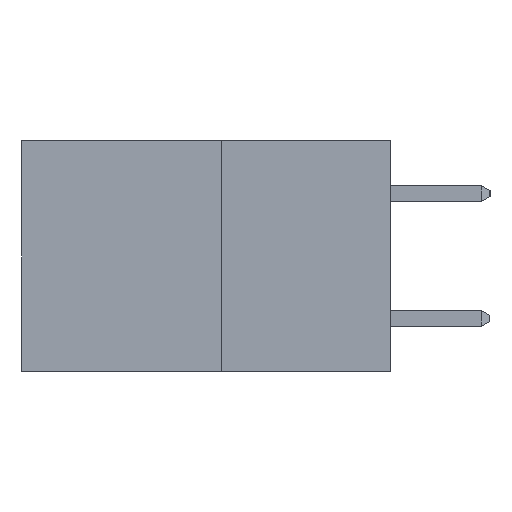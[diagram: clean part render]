
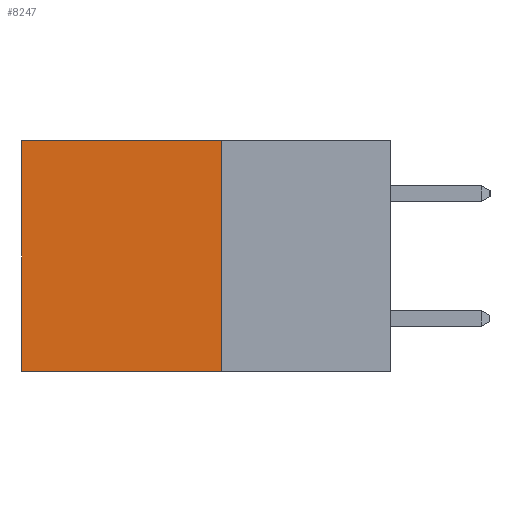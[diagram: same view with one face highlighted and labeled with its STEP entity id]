
A CAD part, left-side view. The second image highlights one B-rep face of the part: STEP entity #8247.
In plain terms, the highlighted planar face has unit normal (-1, 0, 0).
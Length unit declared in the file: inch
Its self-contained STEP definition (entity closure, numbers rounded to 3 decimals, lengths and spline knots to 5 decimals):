
#1089 = CARTESIAN_POINT ( 'NONE',  ( 0.277, 0.27, -0.37 ) ) ;
#1847 = FACE_OUTER_BOUND ( 'NONE', #21281, .T. ) ;
#1925 = EDGE_CURVE ( 'NONE', #2921, #8622, #12004, .T. ) ;
#2556 = EDGE_CURVE ( 'NONE', #2921, #6136, #14029, .T. ) ;
#2921 = VERTEX_POINT ( 'NONE', #9171 ) ;
#3023 = LINE ( 'NONE', #23436, #17572 ) ;
#3614 = DIRECTION ( 'NONE',  ( 1., 0., 0. ) ) ;
#3800 = DIRECTION ( 'NONE',  ( 0., 1., 0. ) ) ;
#3917 = VECTOR ( 'NONE', #9567, 39.37008 ) ;
#6136 = VERTEX_POINT ( 'NONE', #6301 ) ;
#6301 = CARTESIAN_POINT ( 'NONE',  ( 0.277, 0.59, 0. ) ) ;
#6983 = VECTOR ( 'NONE', #17974, 39.37008 ) ;
#7414 = VERTEX_POINT ( 'NONE', #19137 ) ;
#8247 = ADVANCED_FACE ( 'NONE', ( #1847 ), #24306, .F. ) ;
#8622 = VERTEX_POINT ( 'NONE', #14500 ) ;
#9171 = CARTESIAN_POINT ( 'NONE',  ( 0.277, 0.27, 0. ) ) ;
#9567 = DIRECTION ( 'NONE',  ( 0., 1., 0. ) ) ;
#9842 = EDGE_CURVE ( 'NONE', #6136, #7414, #3023, .T. ) ;
#9953 = CARTESIAN_POINT ( 'NONE',  ( 0.277, 0.27, 0. ) ) ;
#11117 = ORIENTED_EDGE ( 'NONE', *, *, #9842, .T. ) ;
#11169 = ORIENTED_EDGE ( 'NONE', *, *, #1925, .F. ) ;
#11365 = LINE ( 'NONE', #15182, #21372 ) ;
#12004 = LINE ( 'NONE', #1089, #6983 ) ;
#13105 = CARTESIAN_POINT ( 'NONE',  ( 0.277, 0.27, -0.37 ) ) ;
#14029 = LINE ( 'NONE', #9953, #3917 ) ;
#14114 = DIRECTION ( 'NONE',  ( 0., 0., -1. ) ) ;
#14500 = CARTESIAN_POINT ( 'NONE',  ( 0.277, 0.27, -0.37 ) ) ;
#15182 = CARTESIAN_POINT ( 'NONE',  ( 0.277, 0.27, -0.37 ) ) ;
#16900 = DIRECTION ( 'NONE',  ( 0., 0., -1. ) ) ;
#17572 = VECTOR ( 'NONE', #14114, 39.37008 ) ;
#17974 = DIRECTION ( 'NONE',  ( 0., 0., -1. ) ) ;
#19137 = CARTESIAN_POINT ( 'NONE',  ( 0.277, 0.59, -0.37 ) ) ;
#19206 = AXIS2_PLACEMENT_3D ( 'NONE', #13105, #3614, #16900 ) ;
#20119 = ORIENTED_EDGE ( 'NONE', *, *, #20873, .F. ) ;
#20873 = EDGE_CURVE ( 'NONE', #8622, #7414, #11365, .T. ) ;
#21197 = ORIENTED_EDGE ( 'NONE', *, *, #2556, .T. ) ;
#21281 = EDGE_LOOP ( 'NONE', ( #11117, #20119, #11169, #21197 ) ) ;
#21372 = VECTOR ( 'NONE', #3800, 39.37008 ) ;
#23436 = CARTESIAN_POINT ( 'NONE',  ( 0.277, 0.59, -0.37 ) ) ;
#24306 = PLANE ( 'NONE',  #19206 ) ;
